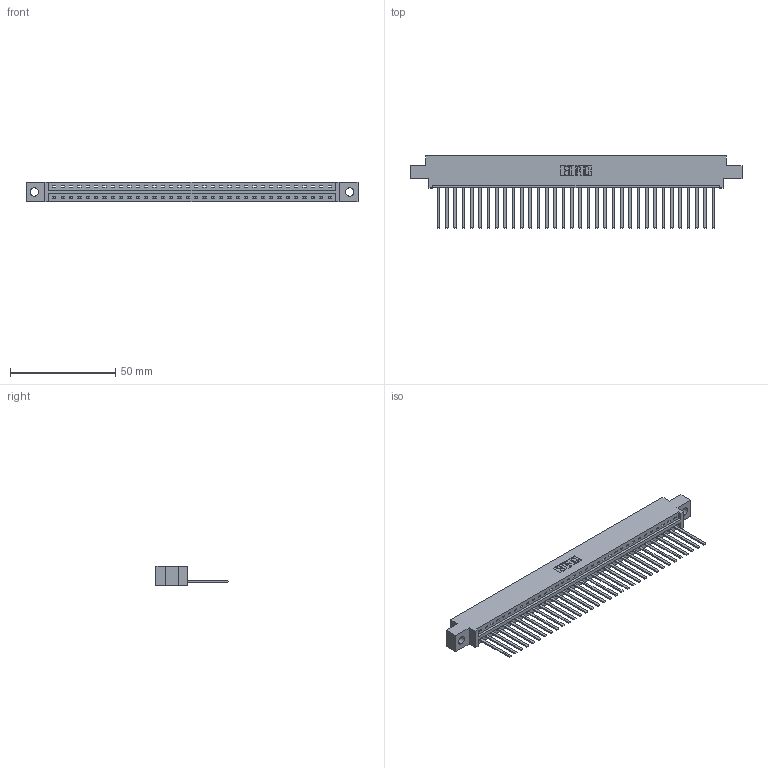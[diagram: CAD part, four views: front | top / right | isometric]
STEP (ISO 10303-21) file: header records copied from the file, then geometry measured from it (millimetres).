
FILE_DESCRIPTION (( 'STEP AP203' ), '1' );
FILE_NAME ('387-034-544-604.STEP', '2019-10-04T11:35:46', ( '' ), ( '' ), 'SwSTEP 2.0', 'SolidWorks 2016', '' );
FILE_SCHEMA (( 'CONFIG_CONTROL_DESIGN' ));
Length unit declared in the file: inch
Products named in the file (3): 345-292-001_345-293-144; 337 Part_0.170 Offset - 0.156 Dia-TH; 387-034-544-604
Assembly tree (35 placements, depth 2):
  387-034-544-604
    337 Part_0.170 Offset - 0.156 Dia-TH
    345-292-001_345-293-144  x34
Bounding box: 157.73 x 34.3 x 9.4 mm (x, y, z)
Volume: 16482.1 mm3; surface area: 18174.4 mm2
Topology: 35 solids, 35 shells, 2022 faces, 6103 edges, 4022 vertices
Faces by surface type: plane 1502, cylinder 520
Entity records: 26259 total; most frequent: CARTESIAN_POINT 4580, ORIENTED_EDGE 4550, DIRECTION 3867, EDGE_CURVE 2275, VECTOR 2151, LINE 2151, VERTEX_POINT 1514, AXIS2_PLACEMENT_3D 858
